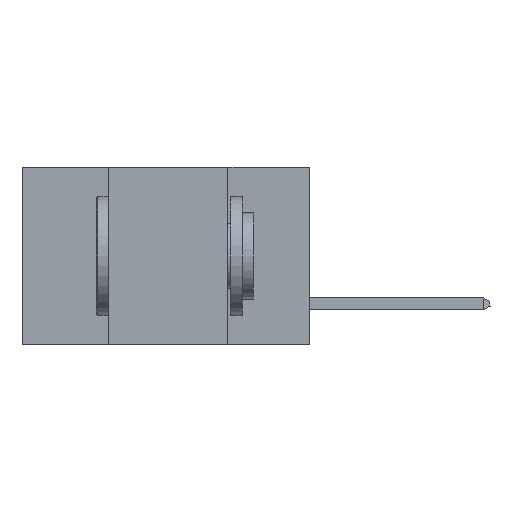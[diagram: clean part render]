
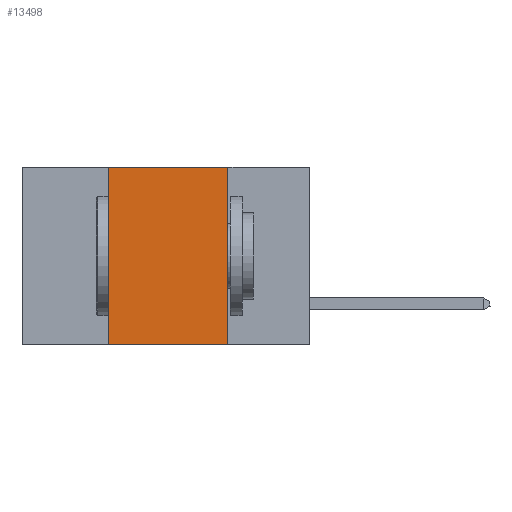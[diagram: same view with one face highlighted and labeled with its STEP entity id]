
A CAD part, left-side view. The second image highlights one B-rep face of the part: STEP entity #13498.
In plain terms, the highlighted planar face has unit normal (-1, 0, 0).
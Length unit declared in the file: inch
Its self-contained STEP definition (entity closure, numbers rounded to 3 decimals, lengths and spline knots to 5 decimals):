
#179 = LINE ( 'NONE', #3126, #32375 ) ;
#971 = VERTEX_POINT ( 'NONE', #10594 ) ;
#1405 = LINE ( 'NONE', #3449, #3255 ) ;
#3126 = CARTESIAN_POINT ( 'NONE',  ( 0., 0.17, 0. ) ) ;
#3255 = VECTOR ( 'NONE', #14381, 39.37008 ) ;
#3449 = CARTESIAN_POINT ( 'NONE',  ( 0., 0.42, 0. ) ) ;
#3475 = VERTEX_POINT ( 'NONE', #38480 ) ;
#4810 = EDGE_CURVE ( 'NONE', #3475, #26499, #1405, .T. ) ;
#6562 = ORIENTED_EDGE ( 'NONE', *, *, #27122, .F. ) ;
#6908 = FACE_OUTER_BOUND ( 'NONE', #46913, .T. ) ;
#10594 = CARTESIAN_POINT ( 'NONE',  ( 0., 0.17, -0.37 ) ) ;
#13098 = CARTESIAN_POINT ( 'NONE',  ( 0., 0.42, 0. ) ) ;
#13498 = ADVANCED_FACE ( 'NONE', ( #6908 ), #19316, .F. ) ;
#14061 = DIRECTION ( 'NONE',  ( 0., 0., -1. ) ) ;
#14381 = DIRECTION ( 'NONE',  ( 0., 0., 1. ) ) ;
#16220 = EDGE_CURVE ( 'NONE', #3475, #971, #41593, .T. ) ;
#16500 = EDGE_CURVE ( 'NONE', #26499, #45883, #25873, .T. ) ;
#19316 = PLANE ( 'NONE',  #38659 ) ;
#20834 = DIRECTION ( 'NONE',  ( 0., 0., -1. ) ) ;
#21149 = ORIENTED_EDGE ( 'NONE', *, *, #16220, .T. ) ;
#22053 = CARTESIAN_POINT ( 'NONE',  ( 0., 0.6, 0. ) ) ;
#25492 = DIRECTION ( 'NONE',  ( 0., -1., 0. ) ) ;
#25503 = DIRECTION ( 'NONE',  ( 0., -1., 0. ) ) ;
#25873 = LINE ( 'NONE', #22053, #42736 ) ;
#26499 = VERTEX_POINT ( 'NONE', #13098 ) ;
#27122 = EDGE_CURVE ( 'NONE', #45883, #971, #179, .T. ) ;
#32375 = VECTOR ( 'NONE', #14061, 39.37008 ) ;
#33327 = CARTESIAN_POINT ( 'NONE',  ( 0., 0.6, -0.37 ) ) ;
#34182 = ORIENTED_EDGE ( 'NONE', *, *, #4810, .F. ) ;
#38480 = CARTESIAN_POINT ( 'NONE',  ( 0., 0.42, -0.37 ) ) ;
#38659 = AXIS2_PLACEMENT_3D ( 'NONE', #43131, #46399, #20834 ) ;
#41593 = LINE ( 'NONE', #33327, #48168 ) ;
#42736 = VECTOR ( 'NONE', #25492, 39.37008 ) ;
#43131 = CARTESIAN_POINT ( 'NONE',  ( 0., 0.6, 0. ) ) ;
#45149 = ORIENTED_EDGE ( 'NONE', *, *, #16500, .F. ) ;
#45883 = VERTEX_POINT ( 'NONE', #47720 ) ;
#46399 = DIRECTION ( 'NONE',  ( 1., 0., 0. ) ) ;
#46913 = EDGE_LOOP ( 'NONE', ( #6562, #45149, #34182, #21149 ) ) ;
#47720 = CARTESIAN_POINT ( 'NONE',  ( 0., 0.17, 0. ) ) ;
#48168 = VECTOR ( 'NONE', #25503, 39.37008 ) ;
